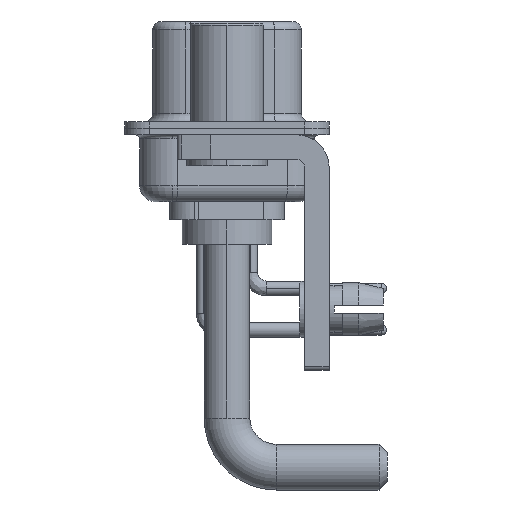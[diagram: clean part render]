
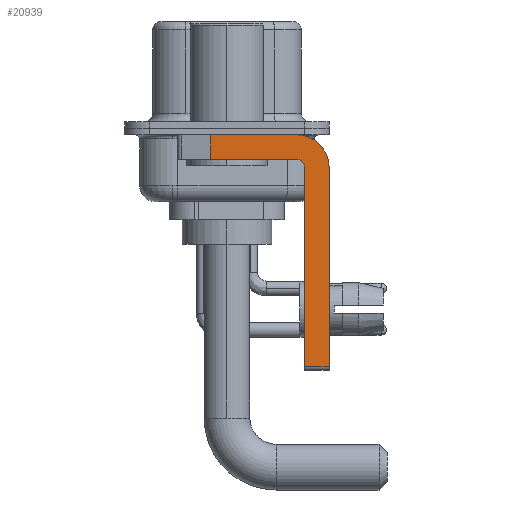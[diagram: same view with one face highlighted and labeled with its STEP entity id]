
A CAD part, left-side view. The second image highlights one B-rep face of the part: STEP entity #20939.
In plain terms, the highlighted planar face has unit normal (-1, 0, 0).
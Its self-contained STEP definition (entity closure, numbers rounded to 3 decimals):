
#44 = DIRECTION ( 'NONE',  ( 0., 0., -1. ) ) ;
#516 = EDGE_CURVE ( 'NONE', #1617, #27236, #19564, .T. ) ;
#728 = EDGE_CURVE ( 'NONE', #3870, #18454, #22911, .T. ) ;
#917 = DIRECTION ( 'NONE',  ( 0., 0., -1. ) ) ;
#1183 = VECTOR ( 'NONE', #12914, 1000. ) ;
#1617 = VERTEX_POINT ( 'NONE', #8509 ) ;
#3333 = CIRCLE ( 'NONE', #19493, 0.5 ) ;
#3870 = VERTEX_POINT ( 'NONE', #8594 ) ;
#4188 = EDGE_CURVE ( 'NONE', #26742, #3870, #7701, .T. ) ;
#4203 = CARTESIAN_POINT ( 'NONE',  ( -2.9, -4.25, -1.9 ) ) ;
#4576 = DIRECTION ( 'NONE',  ( 0., 0., 1. ) ) ;
#5931 = VECTOR ( 'NONE', #23444, 1000. ) ;
#7218 = ORIENTED_EDGE ( 'NONE', *, *, #516, .T. ) ;
#7701 = LINE ( 'NONE', #20577, #17510 ) ;
#7941 = CARTESIAN_POINT ( 'NONE',  ( -2.9, -6.25, -2.4 ) ) ;
#8472 = DIRECTION ( 'NONE',  ( 0., 1., 0. ) ) ;
#8509 = CARTESIAN_POINT ( 'NONE',  ( -2.9, -4.75, -14.55 ) ) ;
#8594 = CARTESIAN_POINT ( 'NONE',  ( -2.9, -4.25, -0.4 ) ) ;
#9004 = CARTESIAN_POINT ( 'NONE',  ( -2.9, -4.25, -2.4 ) ) ;
#9539 = CARTESIAN_POINT ( 'NONE',  ( -2.9, -4.25, -2.4 ) ) ;
#9718 = LINE ( 'NONE', #14473, #10288 ) ;
#10232 = VERTEX_POINT ( 'NONE', #17536 ) ;
#10288 = VECTOR ( 'NONE', #917, 1000. ) ;
#10654 = CARTESIAN_POINT ( 'NONE',  ( -2.9, -4.75, -14.8 ) ) ;
#10976 = EDGE_CURVE ( 'NONE', #18151, #10232, #28321, .T. ) ;
#11226 = LINE ( 'NONE', #10654, #26176 ) ;
#11330 = CARTESIAN_POINT ( 'NONE',  ( -2.9, -6.25, -14.55 ) ) ;
#11431 = ORIENTED_EDGE ( 'NONE', *, *, #728, .F. ) ;
#11443 = VERTEX_POINT ( 'NONE', #25531 ) ;
#12422 = CARTESIAN_POINT ( 'NONE',  ( -2.9, -6.25, -2.4 ) ) ;
#12914 = DIRECTION ( 'NONE',  ( 0., -1., 0. ) ) ;
#14010 = PLANE ( 'NONE',  #21008 ) ;
#14473 = CARTESIAN_POINT ( 'NONE',  ( -2.9, 0.978, -1.9 ) ) ;
#14854 = ORIENTED_EDGE ( 'NONE', *, *, #19130, .T. ) ;
#15060 = ORIENTED_EDGE ( 'NONE', *, *, #18450, .F. ) ;
#16514 = DIRECTION ( 'NONE',  ( 0., -1., 0. ) ) ;
#17510 = VECTOR ( 'NONE', #16514, 1000. ) ;
#17536 = CARTESIAN_POINT ( 'NONE',  ( -2.9, 0.978, -1.9 ) ) ;
#18151 = VERTEX_POINT ( 'NONE', #4203 ) ;
#18450 = EDGE_CURVE ( 'NONE', #11443, #18151, #3333, .T. ) ;
#18454 = VERTEX_POINT ( 'NONE', #7941 ) ;
#18976 = EDGE_LOOP ( 'NONE', ( #28319, #14854, #23272, #15060, #21337, #7218, #27947, #11431 ) ) ;
#19130 = EDGE_CURVE ( 'NONE', #26742, #10232, #9718, .T. ) ;
#19202 = DIRECTION ( 'NONE',  ( -1., 0., 0. ) ) ;
#19493 = AXIS2_PLACEMENT_3D ( 'NONE', #27639, #19202, #21103 ) ;
#19564 = LINE ( 'NONE', #26116, #1183 ) ;
#19770 = CARTESIAN_POINT ( 'NONE',  ( -2.9, 0.978, -0.4 ) ) ;
#19855 = DIRECTION ( 'NONE',  ( 1., 0., 0. ) ) ;
#20577 = CARTESIAN_POINT ( 'NONE',  ( -2.9, 3., -0.4 ) ) ;
#20939 = ADVANCED_FACE ( 'NONE', ( #25332 ), #14010, .F. ) ;
#21008 = AXIS2_PLACEMENT_3D ( 'NONE', #9539, #27222, #26932 ) ;
#21103 = DIRECTION ( 'NONE',  ( 0., 0., 1. ) ) ;
#21206 = CARTESIAN_POINT ( 'NONE',  ( -2.9, -4.25, -1.9 ) ) ;
#21337 = ORIENTED_EDGE ( 'NONE', *, *, #22952, .F. ) ;
#21515 = AXIS2_PLACEMENT_3D ( 'NONE', #9004, #19855, #44 ) ;
#22911 = CIRCLE ( 'NONE', #21515, 2. ) ;
#22952 = EDGE_CURVE ( 'NONE', #1617, #11443, #11226, .T. ) ;
#23272 = ORIENTED_EDGE ( 'NONE', *, *, #10976, .F. ) ;
#23444 = DIRECTION ( 'NONE',  ( 0., 0., -1. ) ) ;
#25332 = FACE_OUTER_BOUND ( 'NONE', #18976, .T. ) ;
#25345 = LINE ( 'NONE', #12422, #5931 ) ;
#25531 = CARTESIAN_POINT ( 'NONE',  ( -2.9, -4.75, -2.4 ) ) ;
#25816 = VECTOR ( 'NONE', #8472, 1000. ) ;
#26116 = CARTESIAN_POINT ( 'NONE',  ( -2.9, -4.25, -14.55 ) ) ;
#26176 = VECTOR ( 'NONE', #4576, 1000. ) ;
#26742 = VERTEX_POINT ( 'NONE', #19770 ) ;
#26932 = DIRECTION ( 'NONE',  ( 0., 0., -1. ) ) ;
#27222 = DIRECTION ( 'NONE',  ( 1., 0., 0. ) ) ;
#27236 = VERTEX_POINT ( 'NONE', #11330 ) ;
#27397 = EDGE_CURVE ( 'NONE', #18454, #27236, #25345, .T. ) ;
#27639 = CARTESIAN_POINT ( 'NONE',  ( -2.9, -4.25, -2.4 ) ) ;
#27947 = ORIENTED_EDGE ( 'NONE', *, *, #27397, .F. ) ;
#28319 = ORIENTED_EDGE ( 'NONE', *, *, #4188, .F. ) ;
#28321 = LINE ( 'NONE', #21206, #25816 ) ;
